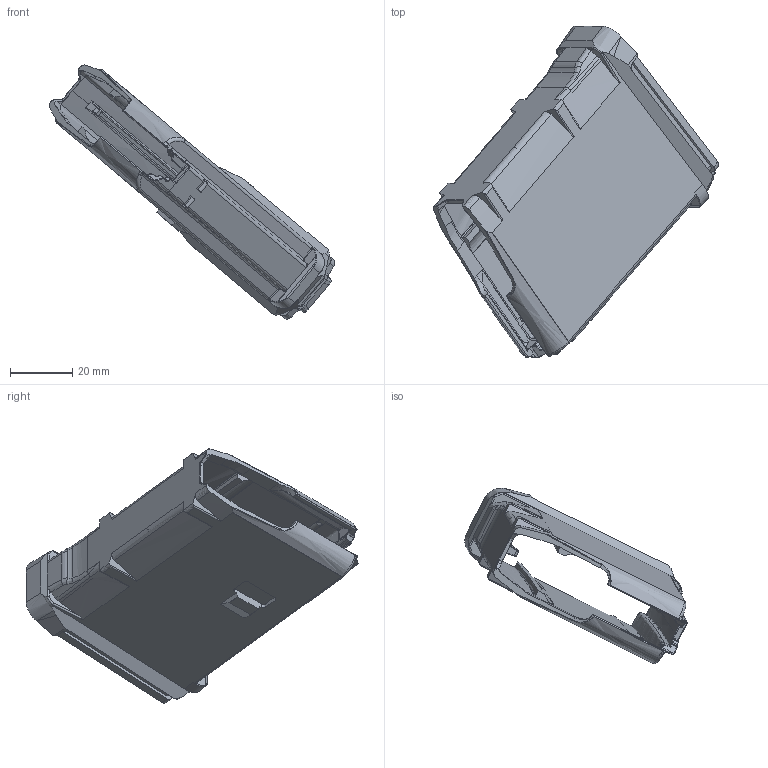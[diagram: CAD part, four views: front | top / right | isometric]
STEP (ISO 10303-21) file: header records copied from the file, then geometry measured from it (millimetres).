
FILE_DESCRIPTION (( 'STEP AP214' ), '1' );
FILE_NAME ('10rd_Base.STEP', '2022-09-24T15:45:06', ( '' ), ( '' ), 'SwSTEP 2.0', 'SolidWorks 2021', '' );
FILE_SCHEMA (( 'AUTOMOTIVE_DESIGN' ));
Length unit declared in the file: millimetre
Products named in the file (1): 10rd_Base
Bounding box: 91.56 x 106.39 x 81.43 mm (x, y, z)
Volume: 30223.5 mm3; surface area: 29793 mm2
Topology: 1 solids, 2 shells, 579 faces, 1535 edges, 958 vertices
Faces by surface type: bspline 289, plane 180, cylinder 100, sphere 6, torus 4
Entity records: 29281 total; most frequent: CARTESIAN_POINT 17715, ORIENTED_EDGE 3066, EDGE_CURVE 1533, DIRECTION 1415, VERTEX_POINT 958, B_SPLINE_CURVE_WITH_KNOTS 758, EDGE_LOOP 581, ADVANCED_FACE 579
